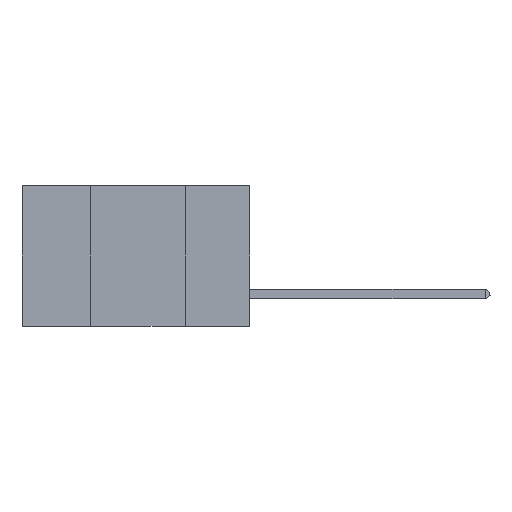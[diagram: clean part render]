
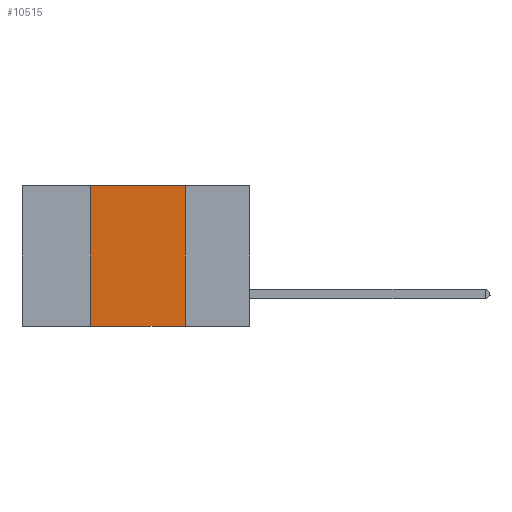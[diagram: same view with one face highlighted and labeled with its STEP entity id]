
A CAD part, left-side view. The second image highlights one B-rep face of the part: STEP entity #10515.
In plain terms, the highlighted planar face has unit normal (-1, 0, 0).
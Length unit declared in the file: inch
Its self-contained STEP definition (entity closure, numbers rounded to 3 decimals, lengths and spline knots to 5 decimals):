
#1435 = LINE ( 'NONE', #13957, #6322 ) ;
#1689 = VECTOR ( 'NONE', #11500, 39.37008 ) ;
#1942 = VECTOR ( 'NONE', #4265, 39.37008 ) ;
#2599 = ORIENTED_EDGE ( 'NONE', *, *, #11738, .F. ) ;
#2720 = ORIENTED_EDGE ( 'NONE', *, *, #13686, .F. ) ;
#3216 = VERTEX_POINT ( 'NONE', #5021 ) ;
#3287 = EDGE_CURVE ( 'NONE', #11153, #9490, #1435, .T. ) ;
#3742 = DIRECTION ( 'NONE',  ( 0., 0., -1. ) ) ;
#4001 = EDGE_CURVE ( 'NONE', #3216, #9490, #6325, .T. ) ;
#4183 = DIRECTION ( 'NONE',  ( 0., -1., 0. ) ) ;
#4265 = DIRECTION ( 'NONE',  ( 0., 0., 1. ) ) ;
#4510 = LINE ( 'NONE', #8984, #1689 ) ;
#4514 = DIRECTION ( 'NONE',  ( 1., 0., 0. ) ) ;
#4731 = AXIS2_PLACEMENT_3D ( 'NONE', #4872, #4514, #3742 ) ;
#4872 = CARTESIAN_POINT ( 'NONE',  ( 0., 0.6, 0. ) ) ;
#5021 = CARTESIAN_POINT ( 'NONE',  ( 0., 0.42, -0.37 ) ) ;
#6322 = VECTOR ( 'NONE', #11461, 39.37008 ) ;
#6325 = LINE ( 'NONE', #11481, #10899 ) ;
#6603 = CARTESIAN_POINT ( 'NONE',  ( 0., 0.42, 0. ) ) ;
#7159 = ORIENTED_EDGE ( 'NONE', *, *, #4001, .T. ) ;
#8984 = CARTESIAN_POINT ( 'NONE',  ( 0., 0.6, 0. ) ) ;
#9161 = FACE_OUTER_BOUND ( 'NONE', #14281, .T. ) ;
#9490 = VERTEX_POINT ( 'NONE', #14357 ) ;
#9503 = LINE ( 'NONE', #6603, #1942 ) ;
#9573 = CARTESIAN_POINT ( 'NONE',  ( 0., 0.42, 0. ) ) ;
#10515 = ADVANCED_FACE ( 'NONE', ( #9161 ), #15394, .F. ) ;
#10899 = VECTOR ( 'NONE', #4183, 39.37008 ) ;
#11153 = VERTEX_POINT ( 'NONE', #13322 ) ;
#11461 = DIRECTION ( 'NONE',  ( 0., 0., -1. ) ) ;
#11481 = CARTESIAN_POINT ( 'NONE',  ( 0., 0.6, -0.37 ) ) ;
#11500 = DIRECTION ( 'NONE',  ( 0., -1., 0. ) ) ;
#11738 = EDGE_CURVE ( 'NONE', #3216, #15315, #9503, .T. ) ;
#13322 = CARTESIAN_POINT ( 'NONE',  ( 0., 0.17, 0. ) ) ;
#13686 = EDGE_CURVE ( 'NONE', #15315, #11153, #4510, .T. ) ;
#13957 = CARTESIAN_POINT ( 'NONE',  ( 0., 0.17, 0. ) ) ;
#14281 = EDGE_LOOP ( 'NONE', ( #15186, #2720, #2599, #7159 ) ) ;
#14357 = CARTESIAN_POINT ( 'NONE',  ( 0., 0.17, -0.37 ) ) ;
#15186 = ORIENTED_EDGE ( 'NONE', *, *, #3287, .F. ) ;
#15315 = VERTEX_POINT ( 'NONE', #9573 ) ;
#15394 = PLANE ( 'NONE',  #4731 ) ;
